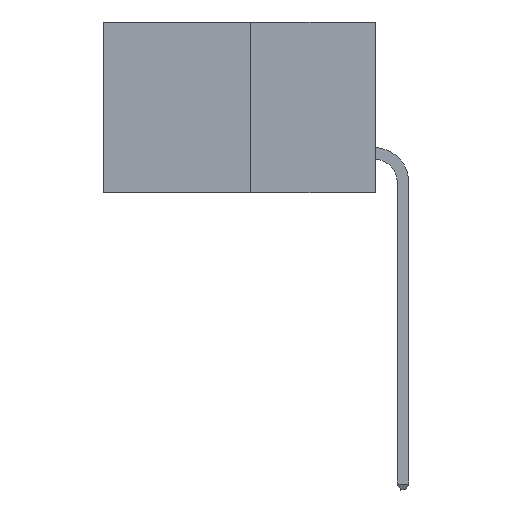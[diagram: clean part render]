
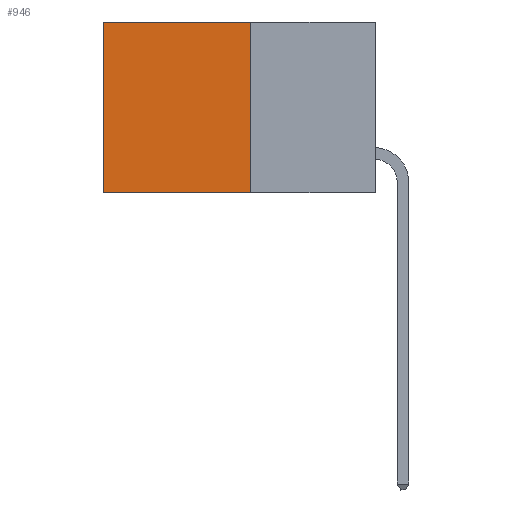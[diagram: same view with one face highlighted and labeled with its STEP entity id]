
A CAD part, left-side view. The second image highlights one B-rep face of the part: STEP entity #946.
In plain terms, the highlighted planar face has unit normal (-1, 0, 0).
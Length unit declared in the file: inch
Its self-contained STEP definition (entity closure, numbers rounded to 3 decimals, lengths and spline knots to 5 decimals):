
#409 = EDGE_CURVE ( 'NONE', #2251, #7782, #6836, .T. ) ;
#476 = EDGE_CURVE ( 'NONE', #5464, #7782, #7479, .T. ) ;
#946 = ADVANCED_FACE ( 'NONE', ( #2332 ), #5437, .F. ) ;
#1262 = CARTESIAN_POINT ( 'NONE',  ( 0.277, 0.27, -0.37 ) ) ;
#1556 = DIRECTION ( 'NONE',  ( 0., 0., -1. ) ) ;
#1569 = CARTESIAN_POINT ( 'NONE',  ( 0.277, 0.27, 0. ) ) ;
#1781 = ORIENTED_EDGE ( 'NONE', *, *, #3675, .F. ) ;
#2017 = EDGE_LOOP ( 'NONE', ( #5331, #5086, #1781, #7181 ) ) ;
#2099 = VECTOR ( 'NONE', #7028, 39.37008 ) ;
#2215 = VERTEX_POINT ( 'NONE', #1569 ) ;
#2251 = VERTEX_POINT ( 'NONE', #4985 ) ;
#2332 = FACE_OUTER_BOUND ( 'NONE', #2017, .T. ) ;
#3285 = CARTESIAN_POINT ( 'NONE',  ( 0.277, 0.27, -0.37 ) ) ;
#3675 = EDGE_CURVE ( 'NONE', #2215, #5464, #4496, .T. ) ;
#3908 = CARTESIAN_POINT ( 'NONE',  ( 0.277, 0.27, 0. ) ) ;
#4008 = EDGE_CURVE ( 'NONE', #2215, #2251, #5755, .T. ) ;
#4496 = LINE ( 'NONE', #1262, #5837 ) ;
#4754 = CARTESIAN_POINT ( 'NONE',  ( 0.277, 0.27, -0.37 ) ) ;
#4985 = CARTESIAN_POINT ( 'NONE',  ( 0.277, 0.59, 0. ) ) ;
#5086 = ORIENTED_EDGE ( 'NONE', *, *, #476, .F. ) ;
#5290 = CARTESIAN_POINT ( 'NONE',  ( 0.277, 0.27, -0.37 ) ) ;
#5331 = ORIENTED_EDGE ( 'NONE', *, *, #409, .T. ) ;
#5420 = DIRECTION ( 'NONE',  ( 0., 1., 0. ) ) ;
#5437 = PLANE ( 'NONE',  #7598 ) ;
#5464 = VERTEX_POINT ( 'NONE', #3285 ) ;
#5575 = VECTOR ( 'NONE', #6234, 39.37008 ) ;
#5755 = LINE ( 'NONE', #3908, #5575 ) ;
#5837 = VECTOR ( 'NONE', #1556, 39.37008 ) ;
#6234 = DIRECTION ( 'NONE',  ( 0., 1., 0. ) ) ;
#6288 = VECTOR ( 'NONE', #5420, 39.37008 ) ;
#6567 = CARTESIAN_POINT ( 'NONE',  ( 0.277, 0.59, -0.37 ) ) ;
#6584 = DIRECTION ( 'NONE',  ( 0., 0., -1. ) ) ;
#6836 = LINE ( 'NONE', #7155, #2099 ) ;
#7028 = DIRECTION ( 'NONE',  ( 0., 0., -1. ) ) ;
#7046 = DIRECTION ( 'NONE',  ( 1., 0., 0. ) ) ;
#7155 = CARTESIAN_POINT ( 'NONE',  ( 0.277, 0.59, -0.37 ) ) ;
#7181 = ORIENTED_EDGE ( 'NONE', *, *, #4008, .T. ) ;
#7479 = LINE ( 'NONE', #5290, #6288 ) ;
#7598 = AXIS2_PLACEMENT_3D ( 'NONE', #4754, #7046, #6584 ) ;
#7782 = VERTEX_POINT ( 'NONE', #6567 ) ;
